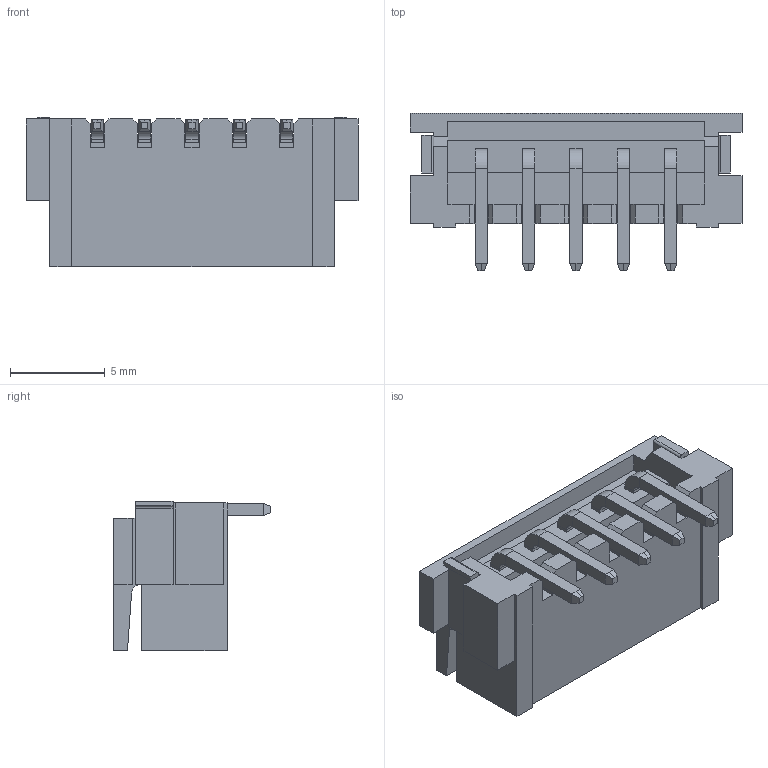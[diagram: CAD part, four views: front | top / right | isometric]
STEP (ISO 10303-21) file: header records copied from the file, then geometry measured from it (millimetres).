
FILE_DESCRIPTION (( 'STEP AP203' ), '1' );
FILE_NAME ('14K-505-418TAA1.STEP', '2024-02-22T14:20:39', ( '' ), ( '' ), 'SwSTEP 2.0', 'SolidWorks 2023', '' );
FILE_SCHEMA (( 'CONFIG_CONTROL_DESIGN' ));
Length unit declared in the file: millimetre
Products named in the file (3): 14K Series SMT Pin_Top Entry; 14K Series SMT Top Entry Insulator_505; 14K-505-418TAA1
Assembly tree (6 placements, depth 2):
  14K-505-418TAA1
    14K Series SMT Top Entry Insulator_505
    14K Series SMT Pin_Top Entry  x5
Bounding box: 17.5 x 8.3 x 7.9 mm (x, y, z)
Volume: 325.7 mm3; surface area: 999.3 mm2
Topology: 6 solids, 6 shells, 302 faces, 772 edges, 482 vertices
Faces by surface type: plane 276, cylinder 26
Entity records: 6895 total; most frequent: CARTESIAN_POINT 1163, ORIENTED_EDGE 1144, DIRECTION 1036, EDGE_CURVE 572, VECTOR 534, LINE 534, VERTEX_POINT 370, AXIS2_PLACEMENT_3D 251
